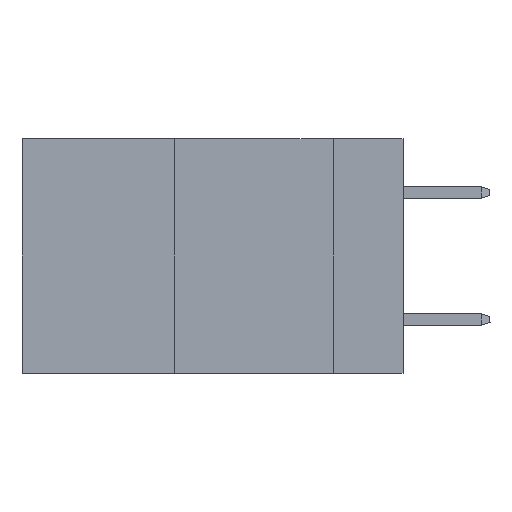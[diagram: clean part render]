
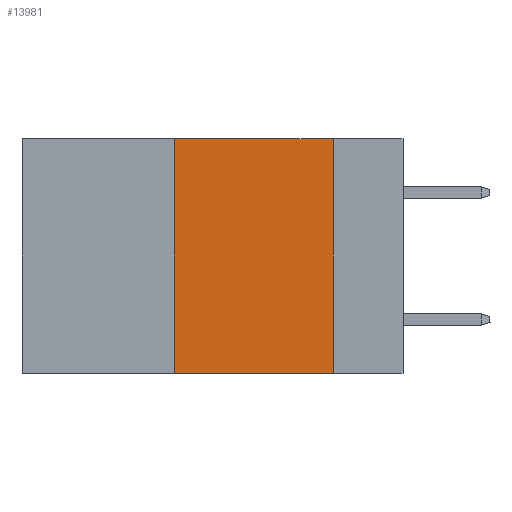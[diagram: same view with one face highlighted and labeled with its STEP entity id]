
A CAD part, left-side view. The second image highlights one B-rep face of the part: STEP entity #13981.
In plain terms, the highlighted planar face has unit normal (-1, 0, 0).
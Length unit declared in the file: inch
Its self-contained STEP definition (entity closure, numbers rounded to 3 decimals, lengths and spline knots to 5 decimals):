
#146 = CARTESIAN_POINT ( 'NONE',  ( 0., 0.11, 0. ) ) ;
#939 = CARTESIAN_POINT ( 'NONE',  ( 0., 0.11, 0. ) ) ;
#1655 = CARTESIAN_POINT ( 'NONE',  ( 0., 0.36, 0. ) ) ;
#1816 = EDGE_CURVE ( 'NONE', #14222, #6217, #6676, .T. ) ;
#1953 = CARTESIAN_POINT ( 'NONE',  ( 0., 0.11, -0.37 ) ) ;
#2066 = VERTEX_POINT ( 'NONE', #1953 ) ;
#2279 = VECTOR ( 'NONE', #4405, 39.37008 ) ;
#2345 = VERTEX_POINT ( 'NONE', #939 ) ;
#2744 = CARTESIAN_POINT ( 'NONE',  ( 0., 0.6, -0.37 ) ) ;
#2963 = FACE_OUTER_BOUND ( 'NONE', #9267, .T. ) ;
#3188 = CARTESIAN_POINT ( 'NONE',  ( 0., 0.36, -0.37 ) ) ;
#3267 = ORIENTED_EDGE ( 'NONE', *, *, #5265, .F. ) ;
#3419 = DIRECTION ( 'NONE',  ( 0., -1., 0. ) ) ;
#4405 = DIRECTION ( 'NONE',  ( 0., 0., 1. ) ) ;
#5265 = EDGE_CURVE ( 'NONE', #2345, #2066, #15369, .T. ) ;
#6217 = VERTEX_POINT ( 'NONE', #15225 ) ;
#6231 = LINE ( 'NONE', #2744, #12070 ) ;
#6351 = VECTOR ( 'NONE', #3419, 39.37008 ) ;
#6531 = DIRECTION ( 'NONE',  ( 0., 0., -1. ) ) ;
#6676 = LINE ( 'NONE', #1655, #2279 ) ;
#7445 = AXIS2_PLACEMENT_3D ( 'NONE', #11328, #8777, #6531 ) ;
#7643 = ORIENTED_EDGE ( 'NONE', *, *, #15224, .T. ) ;
#8070 = ORIENTED_EDGE ( 'NONE', *, *, #1816, .F. ) ;
#8539 = CARTESIAN_POINT ( 'NONE',  ( 0., 0.6, 0. ) ) ;
#8632 = DIRECTION ( 'NONE',  ( 0., 0., -1. ) ) ;
#8777 = DIRECTION ( 'NONE',  ( 1., 0., 0. ) ) ;
#9267 = EDGE_LOOP ( 'NONE', ( #3267, #14616, #8070, #7643 ) ) ;
#9940 = EDGE_CURVE ( 'NONE', #6217, #2345, #11013, .T. ) ;
#10056 = PLANE ( 'NONE',  #7445 ) ;
#11013 = LINE ( 'NONE', #8539, #6351 ) ;
#11328 = CARTESIAN_POINT ( 'NONE',  ( 0., 0.6, 0. ) ) ;
#11927 = VECTOR ( 'NONE', #8632, 39.37008 ) ;
#12070 = VECTOR ( 'NONE', #15630, 39.37008 ) ;
#13981 = ADVANCED_FACE ( 'NONE', ( #2963 ), #10056, .F. ) ;
#14222 = VERTEX_POINT ( 'NONE', #3188 ) ;
#14616 = ORIENTED_EDGE ( 'NONE', *, *, #9940, .F. ) ;
#15224 = EDGE_CURVE ( 'NONE', #14222, #2066, #6231, .T. ) ;
#15225 = CARTESIAN_POINT ( 'NONE',  ( 0., 0.36, 0. ) ) ;
#15369 = LINE ( 'NONE', #146, #11927 ) ;
#15630 = DIRECTION ( 'NONE',  ( 0., -1., 0. ) ) ;
